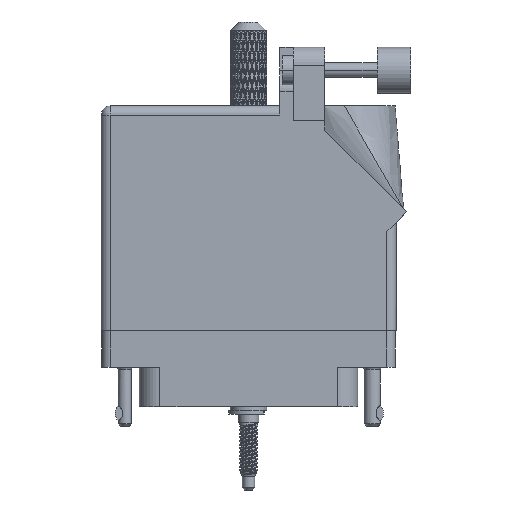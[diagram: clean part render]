
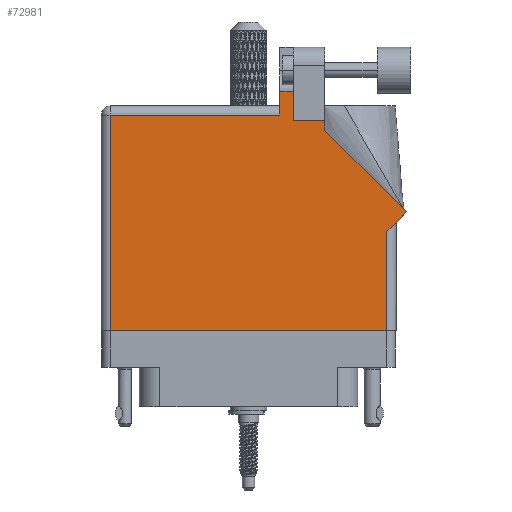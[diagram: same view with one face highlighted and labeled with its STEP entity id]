
A CAD part, front view. The second image highlights one B-rep face of the part: STEP entity #72981.
In plain terms, the highlighted face is planar.
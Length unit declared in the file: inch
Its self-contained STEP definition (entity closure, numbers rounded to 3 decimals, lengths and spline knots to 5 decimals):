
#2659 = VECTOR ( 'NONE', #47466, 39.37008 ) ;
#3035 = CARTESIAN_POINT ( 'NONE',  ( 0.306, 1.5315, 0.455 ) ) ;
#5439 = DIRECTION ( 'NONE',  ( -1., 0., 0. ) ) ;
#6768 = LINE ( 'NONE', #46305, #2659 ) ;
#8377 = ORIENTED_EDGE ( 'NONE', *, *, #9687, .T. ) ;
#9687 = EDGE_CURVE ( 'NONE', #91611, #27298, #22469, .T. ) ;
#10958 = VECTOR ( 'NONE', #17819, 39.37008 ) ;
#12946 = EDGE_CURVE ( 'NONE', #106271, #91611, #85283, .T. ) ;
#14061 = ORIENTED_EDGE ( 'NONE', *, *, #12946, .T. ) ;
#14828 = CARTESIAN_POINT ( 'NONE',  ( 0.519, 1.33, 0.455 ) ) ;
#17393 = CARTESIAN_POINT ( 'NONE',  ( -0.943, -0.1, 0.455 ) ) ;
#17819 = DIRECTION ( 'NONE',  ( -0.707, 0.707, 0. ) ) ;
#19289 = EDGE_CURVE ( 'NONE', #43551, #64980, #110919, .T. ) ;
#20139 = DIRECTION ( 'NONE',  ( 0.707, 0.707, 0. ) ) ;
#20783 = CARTESIAN_POINT ( 'NONE',  ( 0.519, 1.33, 0.455 ) ) ;
#21547 = CARTESIAN_POINT ( 'NONE',  ( 0.212, 1.368, 0.455 ) ) ;
#22469 = LINE ( 'NONE', #61726, #82471 ) ;
#23845 = VECTOR ( 'NONE', #101191, 39.37008 ) ;
#24621 = VECTOR ( 'NONE', #86123, 39.37008 ) ;
#25049 = DIRECTION ( 'NONE',  ( 0., 1., 0. ) ) ;
#25672 = CARTESIAN_POINT ( 'NONE',  ( 0.943, 0.575, 0.455 ) ) ;
#25917 = VECTOR ( 'NONE', #71217, 39.37008 ) ;
#27298 = VERTEX_POINT ( 'NONE', #104334 ) ;
#27936 = LINE ( 'NONE', #20783, #89347 ) ;
#30964 = VERTEX_POINT ( 'NONE', #46148 ) ;
#33376 = CARTESIAN_POINT ( 'NONE',  ( -1.005, -0.1, 0.455 ) ) ;
#33776 = ORIENTED_EDGE ( 'NONE', *, *, #70791, .T. ) ;
#33914 = CARTESIAN_POINT ( 'NONE',  ( 0.519, 1.26442, 0.455 ) ) ;
#34311 = ORIENTED_EDGE ( 'NONE', *, *, #64754, .T. ) ;
#35301 = ORIENTED_EDGE ( 'NONE', *, *, #90975, .T. ) ;
#35947 = CARTESIAN_POINT ( 'NONE',  ( -0.943, 1.368, 0.455 ) ) ;
#36885 = ORIENTED_EDGE ( 'NONE', *, *, #37950, .T. ) ;
#37950 = EDGE_CURVE ( 'NONE', #30964, #60390, #39849, .T. ) ;
#39785 = VECTOR ( 'NONE', #42406, 39.37008 ) ;
#39849 = LINE ( 'NONE', #107429, #25917 ) ;
#40379 = VERTEX_POINT ( 'NONE', #90945 ) ;
#42406 = DIRECTION ( 'NONE',  ( -1., 0., 0. ) ) ;
#42422 = EDGE_CURVE ( 'NONE', #87782, #106271, #27936, .T. ) ;
#43551 = VERTEX_POINT ( 'NONE', #21547 ) ;
#46148 = CARTESIAN_POINT ( 'NONE',  ( 0.943, -0.1, 0.455 ) ) ;
#46305 = CARTESIAN_POINT ( 'NONE',  ( 0.212, 1.43, 0.455 ) ) ;
#47171 = VECTOR ( 'NONE', #20139, 39.37008 ) ;
#47466 = DIRECTION ( 'NONE',  ( 0., -1., 0. ) ) ;
#48708 = ORIENTED_EDGE ( 'NONE', *, *, #107412, .T. ) ;
#48977 = VERTEX_POINT ( 'NONE', #17393 ) ;
#57063 = CARTESIAN_POINT ( 'NONE',  ( 1.005, 0.637, 0.455 ) ) ;
#60390 = VERTEX_POINT ( 'NONE', #25672 ) ;
#61233 = VECTOR ( 'NONE', #96193, 39.37008 ) ;
#61333 = DIRECTION ( 'NONE',  ( -1., 0., 0. ) ) ;
#61726 = CARTESIAN_POINT ( 'NONE',  ( 0.63677, 1.5315, 0.455 ) ) ;
#63771 = ORIENTED_EDGE ( 'NONE', *, *, #42422, .T. ) ;
#64754 = EDGE_CURVE ( 'NONE', #60390, #40379, #70893, .T. ) ;
#64863 = ORIENTED_EDGE ( 'NONE', *, *, #110560, .T. ) ;
#64980 = VERTEX_POINT ( 'NONE', #35947 ) ;
#69465 = LINE ( 'NONE', #105867, #10958 ) ;
#70325 = EDGE_LOOP ( 'NONE', ( #14061, #8377, #48708, #80940, #35301, #33776, #36885, #34311, #64863, #89612, #63771 ) ) ;
#70791 = EDGE_CURVE ( 'NONE', #48977, #30964, #104103, .T. ) ;
#70893 = LINE ( 'NONE', #57063, #47171 ) ;
#71217 = DIRECTION ( 'NONE',  ( 0., 1., 0. ) ) ;
#72268 = CARTESIAN_POINT ( 'NONE',  ( 0.306, 1.33, 0.455 ) ) ;
#72981 = ADVANCED_FACE ( 'NONE', ( #73306 ), #76661, .F. ) ;
#73306 = FACE_OUTER_BOUND ( 'NONE', #70325, .T. ) ;
#73532 = VERTEX_POINT ( 'NONE', #33914 ) ;
#74759 = CARTESIAN_POINT ( 'NONE',  ( 0.306, 1.33, 0.455 ) ) ;
#76254 = EDGE_CURVE ( 'NONE', #73532, #87782, #88169, .T. ) ;
#76661 = PLANE ( 'NONE',  #88937 ) ;
#80940 = ORIENTED_EDGE ( 'NONE', *, *, #19289, .T. ) ;
#82471 = VECTOR ( 'NONE', #61333, 39.37008 ) ;
#85283 = LINE ( 'NONE', #74759, #23845 ) ;
#85444 = VECTOR ( 'NONE', #25049, 39.37008 ) ;
#86123 = DIRECTION ( 'NONE',  ( 1., 0., 0. ) ) ;
#86507 = LINE ( 'NONE', #87272, #61233 ) ;
#87272 = CARTESIAN_POINT ( 'NONE',  ( -0.943, -0.1, 0.455 ) ) ;
#87782 = VERTEX_POINT ( 'NONE', #14828 ) ;
#88169 = LINE ( 'NONE', #104540, #85444 ) ;
#88937 = AXIS2_PLACEMENT_3D ( 'NONE', #92991, #103093, #5439 ) ;
#89347 = VECTOR ( 'NONE', #91307, 39.37008 ) ;
#89612 = ORIENTED_EDGE ( 'NONE', *, *, #76254, .T. ) ;
#90945 = CARTESIAN_POINT ( 'NONE',  ( 1.07571, 0.70771, 0.455 ) ) ;
#90975 = EDGE_CURVE ( 'NONE', #64980, #48977, #86507, .T. ) ;
#91307 = DIRECTION ( 'NONE',  ( -1., 0., 0. ) ) ;
#91611 = VERTEX_POINT ( 'NONE', #3035 ) ;
#92991 = CARTESIAN_POINT ( 'NONE',  ( -1.005, 1.43, 0.455 ) ) ;
#96193 = DIRECTION ( 'NONE',  ( 0., -1., 0. ) ) ;
#101191 = DIRECTION ( 'NONE',  ( 0., 1., 0. ) ) ;
#103093 = DIRECTION ( 'NONE',  ( 0., 0., -1. ) ) ;
#104103 = LINE ( 'NONE', #33376, #24621 ) ;
#104334 = CARTESIAN_POINT ( 'NONE',  ( 0.212, 1.5315, 0.455 ) ) ;
#104540 = CARTESIAN_POINT ( 'NONE',  ( 0.519, 1.26442, 0.455 ) ) ;
#105867 = CARTESIAN_POINT ( 'NONE',  ( 1.07571, 0.70771, 0.455 ) ) ;
#106271 = VERTEX_POINT ( 'NONE', #72268 ) ;
#107412 = EDGE_CURVE ( 'NONE', #27298, #43551, #6768, .T. ) ;
#107429 = CARTESIAN_POINT ( 'NONE',  ( 0.943, 0.637, 0.455 ) ) ;
#110560 = EDGE_CURVE ( 'NONE', #40379, #73532, #69465, .T. ) ;
#110919 = LINE ( 'NONE', #114507, #39785 ) ;
#114507 = CARTESIAN_POINT ( 'NONE',  ( -1.005, 1.368, 0.455 ) ) ;
